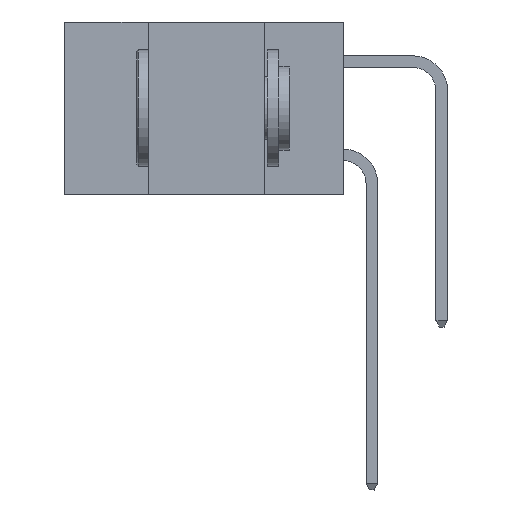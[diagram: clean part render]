
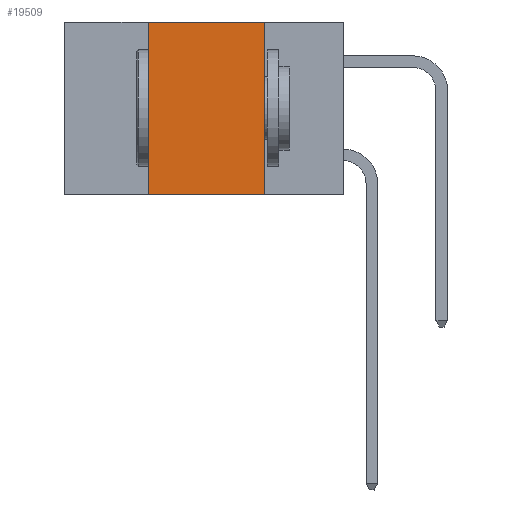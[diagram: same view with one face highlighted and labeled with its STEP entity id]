
A CAD part, left-side view. The second image highlights one B-rep face of the part: STEP entity #19509.
In plain terms, the highlighted planar face has unit normal (-1, 0, 0).
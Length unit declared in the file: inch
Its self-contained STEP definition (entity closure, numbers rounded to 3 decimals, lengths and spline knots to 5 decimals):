
#281 = VERTEX_POINT ( 'NONE', #500 ) ;
#336 = LINE ( 'NONE', #6596, #17705 ) ;
#500 = CARTESIAN_POINT ( 'NONE',  ( 0., 0.17, 0. ) ) ;
#1676 = DIRECTION ( 'NONE',  ( 1., 0., 0. ) ) ;
#2291 = VERTEX_POINT ( 'NONE', #20401 ) ;
#3145 = DIRECTION ( 'NONE',  ( 0., 0., 1. ) ) ;
#3413 = EDGE_CURVE ( 'NONE', #4213, #2291, #21284, .T. ) ;
#4213 = VERTEX_POINT ( 'NONE', #13455 ) ;
#4823 = CARTESIAN_POINT ( 'NONE',  ( 0., 0.6, 0. ) ) ;
#5689 = VERTEX_POINT ( 'NONE', #17405 ) ;
#5920 = ORIENTED_EDGE ( 'NONE', *, *, #9293, .F. ) ;
#6596 = CARTESIAN_POINT ( 'NONE',  ( 0., 0.42, 0. ) ) ;
#6741 = EDGE_LOOP ( 'NONE', ( #16201, #10161, #5920, #17156 ) ) ;
#8465 = CARTESIAN_POINT ( 'NONE',  ( 0., 0.17, 0. ) ) ;
#8514 = CARTESIAN_POINT ( 'NONE',  ( 0., 0.6, -0.37 ) ) ;
#9276 = EDGE_CURVE ( 'NONE', #5689, #281, #9648, .T. ) ;
#9293 = EDGE_CURVE ( 'NONE', #4213, #5689, #336, .T. ) ;
#9648 = LINE ( 'NONE', #4823, #18230 ) ;
#10020 = DIRECTION ( 'NONE',  ( 0., -1., 0. ) ) ;
#10161 = ORIENTED_EDGE ( 'NONE', *, *, #9276, .F. ) ;
#11564 = EDGE_CURVE ( 'NONE', #281, #2291, #16554, .T. ) ;
#11936 = VECTOR ( 'NONE', #22012, 39.37008 ) ;
#12102 = PLANE ( 'NONE',  #13016 ) ;
#12799 = FACE_OUTER_BOUND ( 'NONE', #6741, .T. ) ;
#13016 = AXIS2_PLACEMENT_3D ( 'NONE', #17224, #1676, #13855 ) ;
#13455 = CARTESIAN_POINT ( 'NONE',  ( 0., 0.42, -0.37 ) ) ;
#13855 = DIRECTION ( 'NONE',  ( 0., 0., -1. ) ) ;
#16201 = ORIENTED_EDGE ( 'NONE', *, *, #11564, .F. ) ;
#16554 = LINE ( 'NONE', #8465, #11936 ) ;
#17156 = ORIENTED_EDGE ( 'NONE', *, *, #3413, .T. ) ;
#17224 = CARTESIAN_POINT ( 'NONE',  ( 0., 0.6, 0. ) ) ;
#17405 = CARTESIAN_POINT ( 'NONE',  ( 0., 0.42, 0. ) ) ;
#17705 = VECTOR ( 'NONE', #3145, 39.37008 ) ;
#18230 = VECTOR ( 'NONE', #10020, 39.37008 ) ;
#19509 = ADVANCED_FACE ( 'NONE', ( #12799 ), #12102, .F. ) ;
#20401 = CARTESIAN_POINT ( 'NONE',  ( 0., 0.17, -0.37 ) ) ;
#21284 = LINE ( 'NONE', #8514, #21792 ) ;
#21792 = VECTOR ( 'NONE', #22168, 39.37008 ) ;
#22012 = DIRECTION ( 'NONE',  ( 0., 0., -1. ) ) ;
#22168 = DIRECTION ( 'NONE',  ( 0., -1., 0. ) ) ;
